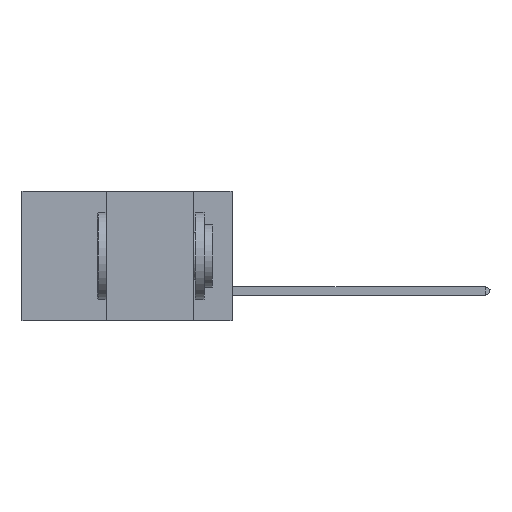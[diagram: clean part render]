
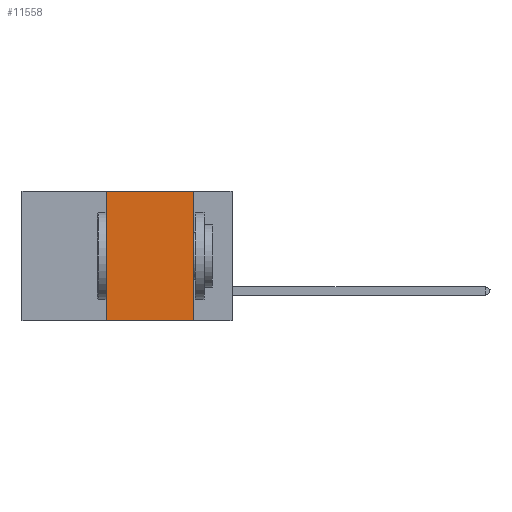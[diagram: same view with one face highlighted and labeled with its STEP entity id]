
A CAD part, left-side view. The second image highlights one B-rep face of the part: STEP entity #11558.
In plain terms, the highlighted planar face has unit normal (-1, 0, 0).
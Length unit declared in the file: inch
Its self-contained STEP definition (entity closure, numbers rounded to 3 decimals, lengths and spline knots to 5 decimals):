
#628 = LINE ( 'NONE', #7363, #13117 ) ;
#2721 = ORIENTED_EDGE ( 'NONE', *, *, #18708, .F. ) ;
#2905 = CARTESIAN_POINT ( 'NONE',  ( 0., 0.11, -0.37 ) ) ;
#3106 = VECTOR ( 'NONE', #9261, 39.37008 ) ;
#3164 = LINE ( 'NONE', #7897, #4637 ) ;
#3487 = EDGE_CURVE ( 'NONE', #10505, #13370, #3164, .T. ) ;
#3536 = VERTEX_POINT ( 'NONE', #15861 ) ;
#4637 = VECTOR ( 'NONE', #14056, 39.37008 ) ;
#5748 = EDGE_LOOP ( 'NONE', ( #17757, #13304, #2721, #15531 ) ) ;
#7363 = CARTESIAN_POINT ( 'NONE',  ( 0., 0.6, 0. ) ) ;
#7604 = VECTOR ( 'NONE', #15615, 39.37008 ) ;
#7672 = CARTESIAN_POINT ( 'NONE',  ( 0., 0.6, 0. ) ) ;
#7813 = DIRECTION ( 'NONE',  ( 1., 0., 0. ) ) ;
#7897 = CARTESIAN_POINT ( 'NONE',  ( 0., 0.6, -0.37 ) ) ;
#8247 = CARTESIAN_POINT ( 'NONE',  ( 0., 0.36, 0. ) ) ;
#8366 = LINE ( 'NONE', #16642, #3106 ) ;
#8937 = CARTESIAN_POINT ( 'NONE',  ( 0., 0.36, -0.37 ) ) ;
#9261 = DIRECTION ( 'NONE',  ( 0., 0., -1. ) ) ;
#10505 = VERTEX_POINT ( 'NONE', #8937 ) ;
#11558 = ADVANCED_FACE ( 'NONE', ( #19340 ), #16869, .F. ) ;
#12887 = LINE ( 'NONE', #15820, #7604 ) ;
#13117 = VECTOR ( 'NONE', #14958, 39.37008 ) ;
#13304 = ORIENTED_EDGE ( 'NONE', *, *, #17432, .F. ) ;
#13370 = VERTEX_POINT ( 'NONE', #2905 ) ;
#14056 = DIRECTION ( 'NONE',  ( 0., -1., 0. ) ) ;
#14958 = DIRECTION ( 'NONE',  ( 0., -1., 0. ) ) ;
#15531 = ORIENTED_EDGE ( 'NONE', *, *, #3487, .T. ) ;
#15615 = DIRECTION ( 'NONE',  ( 0., 0., 1. ) ) ;
#15820 = CARTESIAN_POINT ( 'NONE',  ( 0., 0.36, 0. ) ) ;
#15861 = CARTESIAN_POINT ( 'NONE',  ( 0., 0.11, 0. ) ) ;
#16053 = EDGE_CURVE ( 'NONE', #3536, #13370, #8366, .T. ) ;
#16642 = CARTESIAN_POINT ( 'NONE',  ( 0., 0.11, 0. ) ) ;
#16715 = VERTEX_POINT ( 'NONE', #8247 ) ;
#16869 = PLANE ( 'NONE',  #18661 ) ;
#17432 = EDGE_CURVE ( 'NONE', #16715, #3536, #628, .T. ) ;
#17757 = ORIENTED_EDGE ( 'NONE', *, *, #16053, .F. ) ;
#18395 = DIRECTION ( 'NONE',  ( 0., 0., -1. ) ) ;
#18661 = AXIS2_PLACEMENT_3D ( 'NONE', #7672, #7813, #18395 ) ;
#18708 = EDGE_CURVE ( 'NONE', #10505, #16715, #12887, .T. ) ;
#19340 = FACE_OUTER_BOUND ( 'NONE', #5748, .T. ) ;
